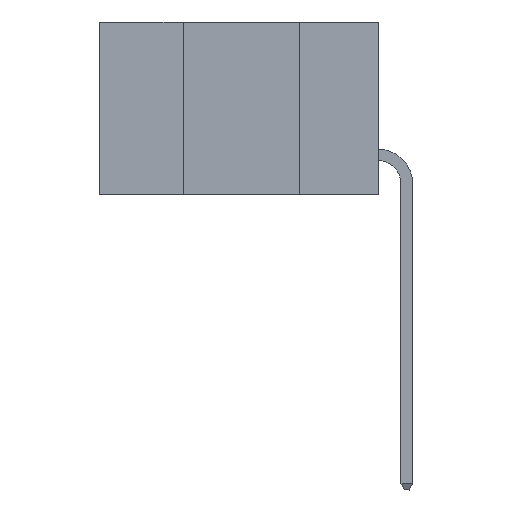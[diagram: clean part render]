
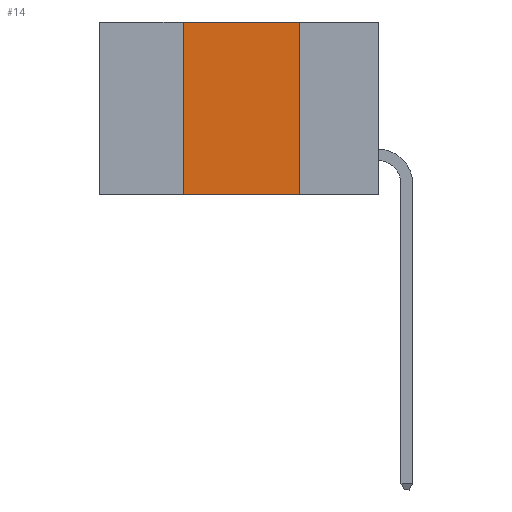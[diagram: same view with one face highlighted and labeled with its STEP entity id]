
A CAD part, left-side view. The second image highlights one B-rep face of the part: STEP entity #14.
In plain terms, the highlighted planar face has unit normal (-1, 0, 0).
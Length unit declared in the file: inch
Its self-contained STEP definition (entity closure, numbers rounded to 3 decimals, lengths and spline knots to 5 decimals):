
#14 = ADVANCED_FACE ( 'NONE', ( #9046 ), #4778, .F. ) ;
#286 = DIRECTION ( 'NONE',  ( 0., 0., -1. ) ) ;
#395 = CARTESIAN_POINT ( 'NONE',  ( 0., 0.17, -0.37 ) ) ;
#845 = VECTOR ( 'NONE', #4335, 39.37008 ) ;
#1096 = CARTESIAN_POINT ( 'NONE',  ( 0., 0.6, 0. ) ) ;
#1106 = DIRECTION ( 'NONE',  ( 0., 0., 1. ) ) ;
#2041 = CARTESIAN_POINT ( 'NONE',  ( 0., 0.17, -0.37 ) ) ;
#2379 = VERTEX_POINT ( 'NONE', #2041 ) ;
#2392 = ORIENTED_EDGE ( 'NONE', *, *, #7768, .T. ) ;
#3018 = ORIENTED_EDGE ( 'NONE', *, *, #8787, .F. ) ;
#3309 = DIRECTION ( 'NONE',  ( 0., -1., 0. ) ) ;
#3793 = VERTEX_POINT ( 'NONE', #4374 ) ;
#4256 = LINE ( 'NONE', #6731, #7177 ) ;
#4335 = DIRECTION ( 'NONE',  ( 0., -1., 0. ) ) ;
#4370 = EDGE_CURVE ( 'NONE', #3793, #2379, #8334, .T. ) ;
#4374 = CARTESIAN_POINT ( 'NONE',  ( 0., 0.17, 0. ) ) ;
#4778 = PLANE ( 'NONE',  #9818 ) ;
#4930 = CARTESIAN_POINT ( 'NONE',  ( 0., 0.42, 0. ) ) ;
#5325 = LINE ( 'NONE', #8727, #845 ) ;
#6465 = EDGE_CURVE ( 'NONE', #10821, #3793, #5325, .T. ) ;
#6731 = CARTESIAN_POINT ( 'NONE',  ( 0., 0.6, -0.37 ) ) ;
#7177 = VECTOR ( 'NONE', #3309, 39.37008 ) ;
#7768 = EDGE_CURVE ( 'NONE', #8560, #2379, #4256, .T. ) ;
#7903 = LINE ( 'NONE', #9598, #10786 ) ;
#8118 = EDGE_LOOP ( 'NONE', ( #10410, #8556, #3018, #2392 ) ) ;
#8334 = LINE ( 'NONE', #395, #9152 ) ;
#8556 = ORIENTED_EDGE ( 'NONE', *, *, #6465, .F. ) ;
#8560 = VERTEX_POINT ( 'NONE', #10180 ) ;
#8727 = CARTESIAN_POINT ( 'NONE',  ( 0., 0.6, 0. ) ) ;
#8787 = EDGE_CURVE ( 'NONE', #8560, #10821, #7903, .T. ) ;
#9046 = FACE_OUTER_BOUND ( 'NONE', #8118, .T. ) ;
#9152 = VECTOR ( 'NONE', #286, 39.37008 ) ;
#9598 = CARTESIAN_POINT ( 'NONE',  ( 0., 0.42, -0.37 ) ) ;
#9818 = AXIS2_PLACEMENT_3D ( 'NONE', #1096, #9866, #10782 ) ;
#9866 = DIRECTION ( 'NONE',  ( 1., 0., 0. ) ) ;
#10180 = CARTESIAN_POINT ( 'NONE',  ( 0., 0.42, -0.37 ) ) ;
#10410 = ORIENTED_EDGE ( 'NONE', *, *, #4370, .F. ) ;
#10782 = DIRECTION ( 'NONE',  ( 0., 0., -1. ) ) ;
#10786 = VECTOR ( 'NONE', #1106, 39.37008 ) ;
#10821 = VERTEX_POINT ( 'NONE', #4930 ) ;
